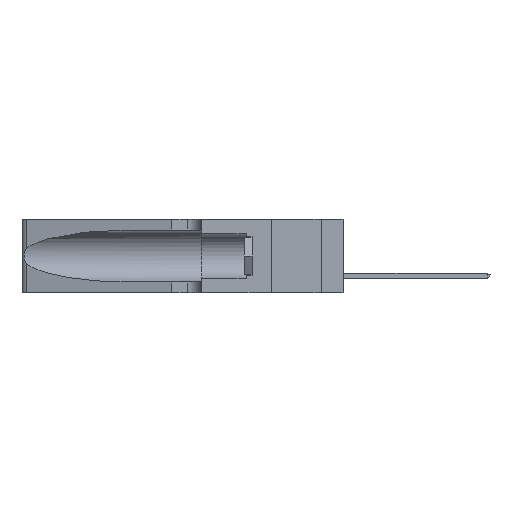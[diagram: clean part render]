
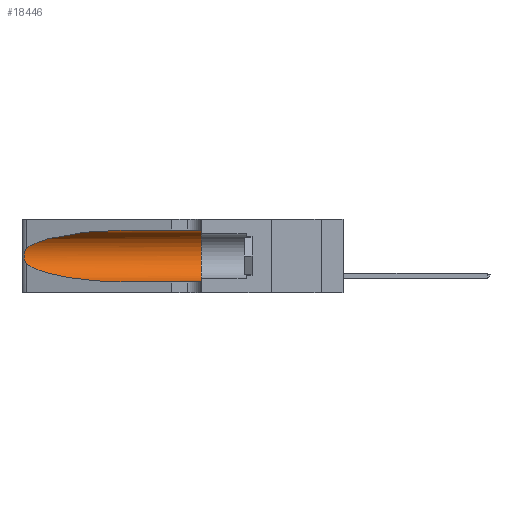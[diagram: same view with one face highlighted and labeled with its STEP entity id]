
A CAD part, left-side view. The second image highlights one B-rep face of the part: STEP entity #18446.
In plain terms, the highlighted cylindrical face has radius 3.308 mm (diameter 6.617 mm), a partial arc.
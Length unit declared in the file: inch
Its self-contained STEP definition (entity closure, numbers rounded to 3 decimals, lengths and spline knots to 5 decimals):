
#747 = DIRECTION ( 'NONE',  ( 0., 0., 1. ) ) ;
#829 = CARTESIAN_POINT ( 'NONE',  ( 0.1305, 0.35, 0.185 ) ) ;
#935 = CARTESIAN_POINT ( 'NONE',  ( 0.25555, 1.22993, 0.14849 ) ) ;
#1012 = CIRCLE ( 'NONE', #15636, 0.13025 ) ;
#1200 = CARTESIAN_POINT ( 'NONE',  ( 0.25854, 1.2359, 0.20912 ) ) ;
#1521 = DIRECTION ( 'NONE',  ( 0., -1., 0. ) ) ;
#1884 = CARTESIAN_POINT ( 'NONE',  ( 0.25487, 1.22718, 0.22369 ) ) ;
#2252 = ORIENTED_EDGE ( 'NONE', *, *, #19627, .F. ) ;
#2352 = VECTOR ( 'NONE', #7434, 39.37008 ) ;
#3026 = CARTESIAN_POINT ( 'NONE',  ( 0.25787, 1.23484, 0.2124 ) ) ;
#3154 = ORIENTED_EDGE ( 'NONE', *, *, #22170, .T. ) ;
#3301 = CARTESIAN_POINT ( 'NONE',  ( 0.1305, 0.35, 0.05475 ) ) ;
#4006 = CARTESIAN_POINT ( 'NONE',  ( 0.1305, 1.61858, 0.185 ) ) ;
#4362 = VERTEX_POINT ( 'NONE', #1884 ) ;
#4595 = ORIENTED_EDGE ( 'NONE', *, *, #8433, .T. ) ;
#4976 = VERTEX_POINT ( 'NONE', #3301 ) ;
#5037 = DIRECTION ( 'NONE',  ( 0., 1., 0. ) ) ;
#5127 = CARTESIAN_POINT ( 'NONE',  ( 0.25856, 1.23593, 0.16098 ) ) ;
#5292 = AXIS2_PLACEMENT_3D ( 'NONE', #4006, #1521, #26985 ) ;
#5314 = CARTESIAN_POINT ( 'NONE',  ( 0.25555, 1.22994, 0.2215 ) ) ;
#5414 = CARTESIAN_POINT ( 'NONE',  ( 0.25487, 1.22718, 0.14631 ) ) ;
#5447 = CARTESIAN_POINT ( 'NONE',  ( 0.2373, 1.15595, 0.08982 ) ) ;
#5767 = EDGE_CURVE ( 'NONE', #23942, #10803, #19290, .T. ) ;
#5957 = EDGE_CURVE ( 'NONE', #15448, #4976, #20256, .T. ) ;
#6315 = ORIENTED_EDGE ( 'NONE', *, *, #5767, .F. ) ;
#6803 =( BOUNDED_CURVE ( )  B_SPLINE_CURVE ( 3, ( #11696, #11602, #26558, #15734 ),
 .UNSPECIFIED., .F., .F. ) 
 B_SPLINE_CURVE_WITH_KNOTS ( ( 4, 4 ),
 ( 1.5708, 2.84003 ),
 .UNSPECIFIED. ) 
 CURVE ( )  GEOMETRIC_REPRESENTATION_ITEM ( )  RATIONAL_B_SPLINE_CURVE ( ( 1., 0.87, 0.87, 1. ) ) 
 REPRESENTATION_ITEM ( '' )  );
#7434 = DIRECTION ( 'NONE',  ( 0., -1., 0. ) ) ;
#7637 = B_SPLINE_CURVE_WITH_KNOTS ( 'NONE', 3,
 ( #22532, #5314, #26454, #3026, #1200, #13570, #9655, #11775, #26729, #5127, #20044, #13752, #935, #24315 ),
 .UNSPECIFIED., .F., .F.,
 ( 4, 2, 2, 2, 2, 2, 4 ),
 ( 0., 0.00027, 0.00053, 0.00107, 0.0016, 0.00187, 0.00214 ),
 .UNSPECIFIED. ) ;
#7976 = EDGE_CURVE ( 'NONE', #17640, #15448, #18732, .T. ) ;
#8433 = EDGE_CURVE ( 'NONE', #23942, #4362, #6803, .T. ) ;
#9312 = FACE_OUTER_BOUND ( 'NONE', #19922, .T. ) ;
#9655 = CARTESIAN_POINT ( 'NONE',  ( 0.26075, 1.23896, 0.19203 ) ) ;
#10803 = VERTEX_POINT ( 'NONE', #12687 ) ;
#11602 = CARTESIAN_POINT ( 'NONE',  ( 0.18966, 0.96281, 0.31525 ) ) ;
#11696 = CARTESIAN_POINT ( 'NONE',  ( 0.1305, 0.72297, 0.31525 ) ) ;
#11775 = CARTESIAN_POINT ( 'NONE',  ( 0.26075, 1.23896, 0.178 ) ) ;
#12687 = CARTESIAN_POINT ( 'NONE',  ( 0.1305, 0.35, 0.31525 ) ) ;
#13570 = CARTESIAN_POINT ( 'NONE',  ( 0.26018, 1.23835, 0.19895 ) ) ;
#13577 = CARTESIAN_POINT ( 'NONE',  ( 0.1305, 0.72297, 0.31525 ) ) ;
#13752 = CARTESIAN_POINT ( 'NONE',  ( 0.25639, 1.23186, 0.15144 ) ) ;
#14800 = CARTESIAN_POINT ( 'NONE',  ( 0.1305, 0.72297, 0.05475 ) ) ;
#15448 = VERTEX_POINT ( 'NONE', #14800 ) ;
#15636 = AXIS2_PLACEMENT_3D ( 'NONE', #829, #5037, #747 ) ;
#15734 = CARTESIAN_POINT ( 'NONE',  ( 0.25487, 1.22718, 0.22369 ) ) ;
#15845 = ORIENTED_EDGE ( 'NONE', *, *, #7976, .T. ) ;
#15884 = DIRECTION ( 'NONE',  ( 0., -1., 0. ) ) ;
#15987 = CARTESIAN_POINT ( 'NONE',  ( 0.1305, 1.61858, 0.05475 ) ) ;
#15991 = CYLINDRICAL_SURFACE ( 'NONE', #5292, 0.13025 ) ;
#16053 = CARTESIAN_POINT ( 'NONE',  ( 0.25487, 1.22718, 0.14631 ) ) ;
#17640 = VERTEX_POINT ( 'NONE', #5414 ) ;
#18446 = ADVANCED_FACE ( 'NONE', ( #9312 ), #15991, .F. ) ;
#18610 = VECTOR ( 'NONE', #15884, 39.37008 ) ;
#18732 =( BOUNDED_CURVE ( )  B_SPLINE_CURVE ( 3, ( #16053, #5447, #22657, #24806 ),
 .UNSPECIFIED., .F., .T. ) 
 B_SPLINE_CURVE_WITH_KNOTS ( ( 4, 4 ),
 ( 3.44316, 4.71239 ),
 .UNSPECIFIED. ) 
 CURVE ( )  GEOMETRIC_REPRESENTATION_ITEM ( )  RATIONAL_B_SPLINE_CURVE ( ( 1., 0.87, 0.87, 1. ) ) 
 REPRESENTATION_ITEM ( '' )  );
#19290 = LINE ( 'NONE', #25773, #18610 ) ;
#19627 = EDGE_CURVE ( 'NONE', #10803, #4976, #1012, .T. ) ;
#19922 = EDGE_LOOP ( 'NONE', ( #4595, #3154, #15845, #22320, #2252, #6315 ) ) ;
#20044 = CARTESIAN_POINT ( 'NONE',  ( 0.25789, 1.23486, 0.15765 ) ) ;
#20256 = LINE ( 'NONE', #15987, #2352 ) ;
#22170 = EDGE_CURVE ( 'NONE', #4362, #17640, #7637, .T. ) ;
#22320 = ORIENTED_EDGE ( 'NONE', *, *, #5957, .T. ) ;
#22532 = CARTESIAN_POINT ( 'NONE',  ( 0.25487, 1.22718, 0.22369 ) ) ;
#22657 = CARTESIAN_POINT ( 'NONE',  ( 0.18966, 0.96281, 0.05475 ) ) ;
#23942 = VERTEX_POINT ( 'NONE', #13577 ) ;
#24315 = CARTESIAN_POINT ( 'NONE',  ( 0.25487, 1.22718, 0.14631 ) ) ;
#24806 = CARTESIAN_POINT ( 'NONE',  ( 0.1305, 0.72297, 0.05475 ) ) ;
#25773 = CARTESIAN_POINT ( 'NONE',  ( 0.1305, 1.61858, 0.31525 ) ) ;
#26454 = CARTESIAN_POINT ( 'NONE',  ( 0.25639, 1.23184, 0.21858 ) ) ;
#26558 = CARTESIAN_POINT ( 'NONE',  ( 0.2373, 1.15595, 0.28018 ) ) ;
#26729 = CARTESIAN_POINT ( 'NONE',  ( 0.26017, 1.23833, 0.17102 ) ) ;
#26985 = DIRECTION ( 'NONE',  ( 0., 0., -1. ) ) ;
